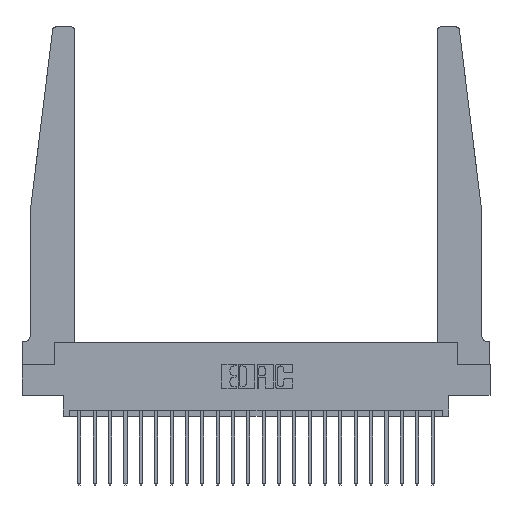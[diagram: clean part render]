
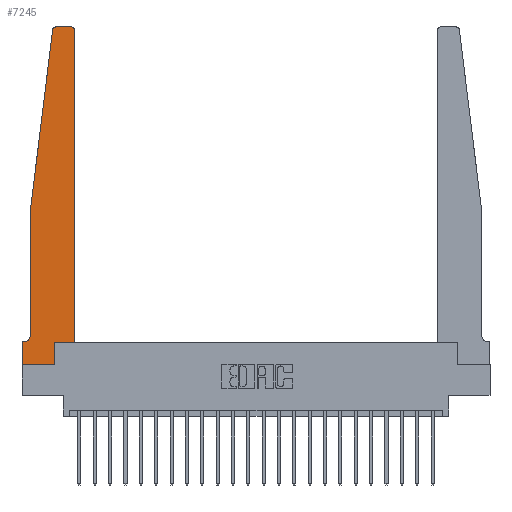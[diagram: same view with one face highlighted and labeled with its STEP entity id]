
A CAD part, top view. The second image highlights one B-rep face of the part: STEP entity #7245.
In plain terms, the highlighted planar face has unit normal (0, 0, 1).
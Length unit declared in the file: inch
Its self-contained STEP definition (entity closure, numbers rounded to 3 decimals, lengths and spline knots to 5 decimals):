
#80 = CARTESIAN_POINT ( 'NONE',  ( 0.065, 0.1875, 0.37 ) ) ;
#132 = LINE ( 'NONE', #7474, #18689 ) ;
#142 = CARTESIAN_POINT ( 'NONE',  ( 0.065, 1.25, 0.37 ) ) ;
#792 = DIRECTION ( 'NONE',  ( 0., -1., 0. ) ) ;
#1008 = CARTESIAN_POINT ( 'NONE',  ( 0., 0., 0.37 ) ) ;
#1617 = CARTESIAN_POINT ( 'NONE',  ( 0.065, 0.2375, 0.37 ) ) ;
#1711 = VERTEX_POINT ( 'NONE', #10532 ) ;
#1747 = VERTEX_POINT ( 'NONE', #17909 ) ;
#1967 = CARTESIAN_POINT ( 'NONE',  ( 0.425, 0.18, 0.37 ) ) ;
#2192 = VECTOR ( 'NONE', #792, 39.37008 ) ;
#2202 = EDGE_CURVE ( 'NONE', #22500, #6462, #12542, .T. ) ;
#2221 = VECTOR ( 'NONE', #21847, 39.37008 ) ;
#2730 = EDGE_CURVE ( 'NONE', #1711, #10651, #18766, .T. ) ;
#2983 = CARTESIAN_POINT ( 'NONE',  ( 0.27653, 2.72, 0.37 ) ) ;
#3001 = EDGE_CURVE ( 'NONE', #17225, #1747, #132, .T. ) ;
#3341 = CARTESIAN_POINT ( 'NONE',  ( 0.2605, 0.18, 0.37 ) ) ;
#3635 = DIRECTION ( 'NONE',  ( -0.122, -0.992, 0. ) ) ;
#3692 = ORIENTED_EDGE ( 'NONE', *, *, #12930, .T. ) ;
#4213 = DIRECTION ( 'NONE',  ( 1., 0., 0. ) ) ;
#4398 = ORIENTED_EDGE ( 'NONE', *, *, #10491, .T. ) ;
#4558 = DIRECTION ( 'NONE',  ( -1., 0., 0. ) ) ;
#4568 = VECTOR ( 'NONE', #20133, 39.37008 ) ;
#4682 = VERTEX_POINT ( 'NONE', #6296 ) ;
#4784 = DIRECTION ( 'NONE',  ( 0., 0., -1. ) ) ;
#4844 = ORIENTED_EDGE ( 'NONE', *, *, #10039, .T. ) ;
#4941 = CIRCLE ( 'NONE', #18203, 0.03 ) ;
#5044 = VECTOR ( 'NONE', #6573, 39.37008 ) ;
#5555 = ORIENTED_EDGE ( 'NONE', *, *, #5789, .T. ) ;
#5691 = AXIS2_PLACEMENT_3D ( 'NONE', #13919, #4784, #4558 ) ;
#5789 = EDGE_CURVE ( 'NONE', #22940, #4682, #17152, .T. ) ;
#6115 = LINE ( 'NONE', #1008, #5044 ) ;
#6296 = CARTESIAN_POINT ( 'NONE',  ( 0., 0., 0.37 ) ) ;
#6462 = VERTEX_POINT ( 'NONE', #142 ) ;
#6573 = DIRECTION ( 'NONE',  ( 1., 0., 0. ) ) ;
#6664 = CARTESIAN_POINT ( 'NONE',  ( 0.395, 2.72, 0.37 ) ) ;
#7245 = ADVANCED_FACE ( 'NONE', ( #8329 ), #21140, .T. ) ;
#7474 = CARTESIAN_POINT ( 'NONE',  ( 0.425, 0.18, 0.37 ) ) ;
#8329 = FACE_OUTER_BOUND ( 'NONE', #13394, .T. ) ;
#8843 = ORIENTED_EDGE ( 'NONE', *, *, #11651, .T. ) ;
#9846 = VERTEX_POINT ( 'NONE', #1617 ) ;
#10039 = EDGE_CURVE ( 'NONE', #9846, #15397, #19733, .T. ) ;
#10337 = CARTESIAN_POINT ( 'NONE',  ( 0.395, 2.75, 0.37 ) ) ;
#10353 = ORIENTED_EDGE ( 'NONE', *, *, #2202, .T. ) ;
#10376 = CARTESIAN_POINT ( 'NONE',  ( 0., 0., 0.37 ) ) ;
#10491 = EDGE_CURVE ( 'NONE', #23231, #22500, #4941, .T. ) ;
#10532 = CARTESIAN_POINT ( 'NONE',  ( 0.2605, 0., 0.37 ) ) ;
#10588 = VERTEX_POINT ( 'NONE', #10337 ) ;
#10612 = CARTESIAN_POINT ( 'NONE',  ( 0.425, 0.18, 0.37 ) ) ;
#10651 = VERTEX_POINT ( 'NONE', #3341 ) ;
#11576 = EDGE_CURVE ( 'NONE', #15397, #22940, #19437, .T. ) ;
#11651 = EDGE_CURVE ( 'NONE', #10651, #17225, #12883, .T. ) ;
#11685 = AXIS2_PLACEMENT_3D ( 'NONE', #6664, #17490, #17612 ) ;
#11815 = ORIENTED_EDGE ( 'NONE', *, *, #11576, .T. ) ;
#12542 = LINE ( 'NONE', #21681, #20248 ) ;
#12664 = DIRECTION ( 'NONE',  ( -1., 0., 0. ) ) ;
#12710 = DIRECTION ( 'NONE',  ( 0., 1., 0. ) ) ;
#12883 = LINE ( 'NONE', #1967, #18550 ) ;
#12886 = CARTESIAN_POINT ( 'NONE',  ( 0.25, 2.75, 0.37 ) ) ;
#12930 = EDGE_CURVE ( 'NONE', #10588, #23231, #18456, .T. ) ;
#12958 = ORIENTED_EDGE ( 'NONE', *, *, #15780, .T. ) ;
#13022 = CARTESIAN_POINT ( 'NONE',  ( 0.27653, 2.75, 0.37 ) ) ;
#13394 = EDGE_LOOP ( 'NONE', ( #3692, #4398, #10353, #20285, #4844, #11815, #5555, #12958, #15518, #8843, #20553, #15866 ) ) ;
#13893 = DIRECTION ( 'NONE',  ( 0., 0., 1. ) ) ;
#13919 = CARTESIAN_POINT ( 'NONE',  ( 0.015, 0.2375, 0.37 ) ) ;
#14145 = CARTESIAN_POINT ( 'NONE',  ( 0., 0.1875, 0.37 ) ) ;
#14703 = LINE ( 'NONE', #19947, #2221 ) ;
#15397 = VERTEX_POINT ( 'NONE', #15864 ) ;
#15518 = ORIENTED_EDGE ( 'NONE', *, *, #2730, .T. ) ;
#15780 = EDGE_CURVE ( 'NONE', #4682, #1711, #6115, .T. ) ;
#15864 = CARTESIAN_POINT ( 'NONE',  ( 0.015, 0.1875, 0.37 ) ) ;
#15866 = ORIENTED_EDGE ( 'NONE', *, *, #20134, .T. ) ;
#16238 = CIRCLE ( 'NONE', #11685, 0.03 ) ;
#17152 = LINE ( 'NONE', #10376, #2192 ) ;
#17225 = VERTEX_POINT ( 'NONE', #10612 ) ;
#17490 = DIRECTION ( 'NONE',  ( 0., 0., 1. ) ) ;
#17612 = DIRECTION ( 'NONE',  ( 1., 0., 0. ) ) ;
#17909 = CARTESIAN_POINT ( 'NONE',  ( 0.425, 2.72, 0.37 ) ) ;
#18203 = AXIS2_PLACEMENT_3D ( 'NONE', #2983, #19126, #20790 ) ;
#18456 = LINE ( 'NONE', #12886, #4568 ) ;
#18549 = AXIS2_PLACEMENT_3D ( 'NONE', #14145, #13893, #21393 ) ;
#18550 = VECTOR ( 'NONE', #4213, 39.37008 ) ;
#18689 = VECTOR ( 'NONE', #12710, 39.37008 ) ;
#18766 = LINE ( 'NONE', #22680, #20005 ) ;
#18879 = DIRECTION ( 'NONE',  ( 0., 1., 0. ) ) ;
#19126 = DIRECTION ( 'NONE',  ( 0., 0., 1. ) ) ;
#19437 = LINE ( 'NONE', #80, #21602 ) ;
#19733 = CIRCLE ( 'NONE', #5691, 0.05 ) ;
#19947 = CARTESIAN_POINT ( 'NONE',  ( 0.065, 1.25, 0.37 ) ) ;
#20005 = VECTOR ( 'NONE', #18879, 39.37008 ) ;
#20133 = DIRECTION ( 'NONE',  ( -1., 0., 0. ) ) ;
#20134 = EDGE_CURVE ( 'NONE', #1747, #10588, #16238, .T. ) ;
#20248 = VECTOR ( 'NONE', #3635, 39.37008 ) ;
#20285 = ORIENTED_EDGE ( 'NONE', *, *, #22941, .T. ) ;
#20553 = ORIENTED_EDGE ( 'NONE', *, *, #3001, .T. ) ;
#20790 = DIRECTION ( 'NONE',  ( 1., 0., 0. ) ) ;
#21140 = PLANE ( 'NONE',  #18549 ) ;
#21393 = DIRECTION ( 'NONE',  ( 1., 0., 0. ) ) ;
#21602 = VECTOR ( 'NONE', #12664, 39.37008 ) ;
#21681 = CARTESIAN_POINT ( 'NONE',  ( 0.065, 1.25, 0.37 ) ) ;
#21847 = DIRECTION ( 'NONE',  ( 0., -1., 0. ) ) ;
#21960 = CARTESIAN_POINT ( 'NONE',  ( 0., 0.1875, 0.37 ) ) ;
#22500 = VERTEX_POINT ( 'NONE', #23190 ) ;
#22680 = CARTESIAN_POINT ( 'NONE',  ( 0.2605, 0.18, 0.37 ) ) ;
#22940 = VERTEX_POINT ( 'NONE', #21960 ) ;
#22941 = EDGE_CURVE ( 'NONE', #6462, #9846, #14703, .T. ) ;
#23190 = CARTESIAN_POINT ( 'NONE',  ( 0.24675, 2.72367, 0.37 ) ) ;
#23231 = VERTEX_POINT ( 'NONE', #13022 ) ;
